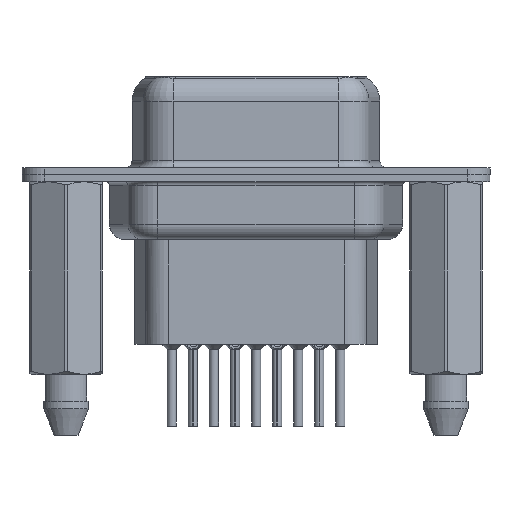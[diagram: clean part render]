
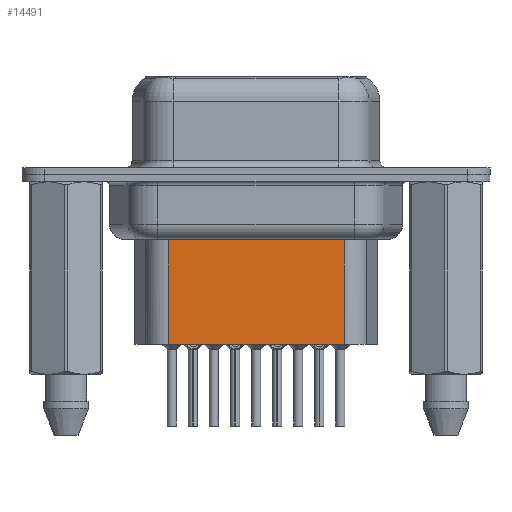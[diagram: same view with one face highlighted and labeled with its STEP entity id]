
A CAD part, front view. The second image highlights one B-rep face of the part: STEP entity #14491.
In plain terms, the highlighted planar face has unit normal (0, -1, 0).
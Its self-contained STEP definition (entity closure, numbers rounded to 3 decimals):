
#1256 = ORIENTED_EDGE ( 'NONE', *, *, #20821, .T. ) ;
#1661 = CARTESIAN_POINT ( 'NONE',  ( 6.706, -3.5, -11.15 ) ) ;
#3196 = VERTEX_POINT ( 'NONE', #19097 ) ;
#3595 = VECTOR ( 'NONE', #17576, 1000. ) ;
#3932 = DIRECTION ( 'NONE',  ( 0., 0., -1. ) ) ;
#4665 = EDGE_CURVE ( 'NONE', #8668, #13798, #14419, .T. ) ;
#5636 = PLANE ( 'NONE',  #5828 ) ;
#5828 = AXIS2_PLACEMENT_3D ( 'NONE', #8995, #15738, #9220 ) ;
#6148 = EDGE_CURVE ( 'NONE', #13798, #16027, #17466, .T. ) ;
#6329 = VECTOR ( 'NONE', #10363, 1000. ) ;
#6408 = CARTESIAN_POINT ( 'NONE',  ( 6.706, -3.5, -3.1 ) ) ;
#6787 = EDGE_LOOP ( 'NONE', ( #13041, #1256, #14651, #20387 ) ) ;
#8668 = VERTEX_POINT ( 'NONE', #9294 ) ;
#8756 = FACE_OUTER_BOUND ( 'NONE', #6787, .T. ) ;
#8995 = CARTESIAN_POINT ( 'NONE',  ( 6.706, -3.5, -3.1 ) ) ;
#9220 = DIRECTION ( 'NONE',  ( 1., 0., 0. ) ) ;
#9294 = CARTESIAN_POINT ( 'NONE',  ( 18.294, -3.5, -4.097 ) ) ;
#10363 = DIRECTION ( 'NONE',  ( -1., 0., 0. ) ) ;
#10589 = CARTESIAN_POINT ( 'NONE',  ( 6.706, -3.5, -11.15 ) ) ;
#12287 = VECTOR ( 'NONE', #3932, 1000. ) ;
#12685 = CARTESIAN_POINT ( 'NONE',  ( 18.294, -3.5, -3.1 ) ) ;
#13041 = ORIENTED_EDGE ( 'NONE', *, *, #4665, .F. ) ;
#13798 = VERTEX_POINT ( 'NONE', #21888 ) ;
#14419 = LINE ( 'NONE', #12685, #12287 ) ;
#14491 = ADVANCED_FACE ( 'NONE', ( #8756 ), #5636, .T. ) ;
#14651 = ORIENTED_EDGE ( 'NONE', *, *, #16457, .T. ) ;
#14702 = VECTOR ( 'NONE', #19344, 1000. ) ;
#15738 = DIRECTION ( 'NONE',  ( 0., -1., 0. ) ) ;
#16027 = VERTEX_POINT ( 'NONE', #1661 ) ;
#16457 = EDGE_CURVE ( 'NONE', #3196, #16027, #22156, .T. ) ;
#17466 = LINE ( 'NONE', #10589, #3595 ) ;
#17576 = DIRECTION ( 'NONE',  ( -1., 0., 0. ) ) ;
#18954 = LINE ( 'NONE', #20806, #6329 ) ;
#19097 = CARTESIAN_POINT ( 'NONE',  ( 6.706, -3.5, -4.097 ) ) ;
#19344 = DIRECTION ( 'NONE',  ( 0., 0., -1. ) ) ;
#20387 = ORIENTED_EDGE ( 'NONE', *, *, #6148, .F. ) ;
#20806 = CARTESIAN_POINT ( 'NONE',  ( 6.459, -3.5, -4.097 ) ) ;
#20821 = EDGE_CURVE ( 'NONE', #8668, #3196, #18954, .T. ) ;
#21888 = CARTESIAN_POINT ( 'NONE',  ( 18.294, -3.5, -11.15 ) ) ;
#22156 = LINE ( 'NONE', #6408, #14702 ) ;
